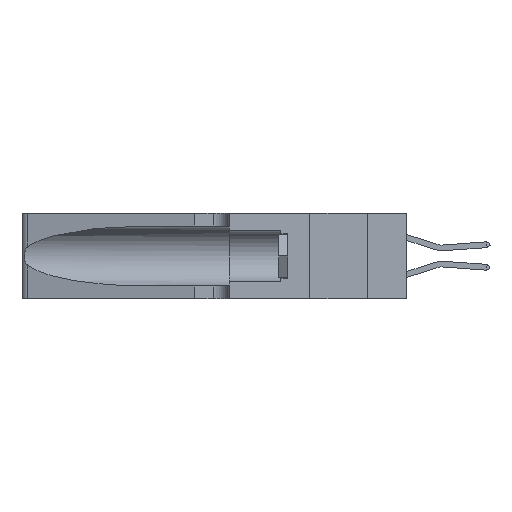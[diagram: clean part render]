
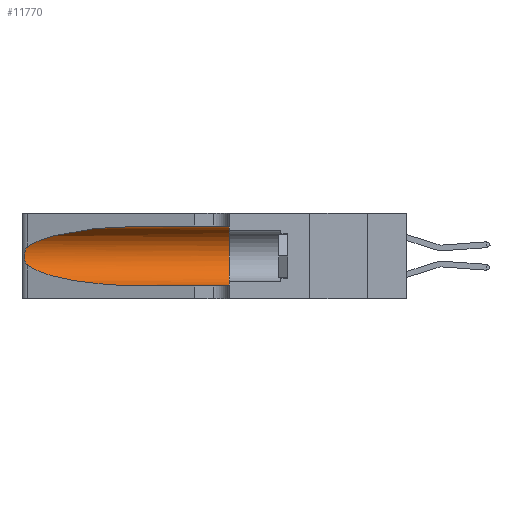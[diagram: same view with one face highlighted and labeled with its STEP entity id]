
A CAD part, left-side view. The second image highlights one B-rep face of the part: STEP entity #11770.
In plain terms, the highlighted cylindrical face has radius 3.308 mm (diameter 6.617 mm), a partial arc.
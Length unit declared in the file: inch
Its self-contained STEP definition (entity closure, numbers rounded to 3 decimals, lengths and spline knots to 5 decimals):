
#532 = AXIS2_PLACEMENT_3D ( 'NONE', #5945, #30028, #9462 ) ;
#824 = CARTESIAN_POINT ( 'NONE',  ( 0.25639, 1.23184, 0.21858 ) ) ;
#1131 = VERTEX_POINT ( 'NONE', #11829 ) ;
#1831 = DIRECTION ( 'NONE',  ( 0., 0., -1. ) ) ;
#1973 = VERTEX_POINT ( 'NONE', #43382 ) ;
#1997 = DIRECTION ( 'NONE',  ( 0., -1., 0. ) ) ;
#2877 = VECTOR ( 'NONE', #40002, 39.37008 ) ;
#3616 = B_SPLINE_CURVE_WITH_KNOTS ( 'NONE', 3,
 ( #18134, #38602, #824, #25039, #4360, #28454, #7872, #31913, #11397, #35346, #14853, #38744, #18292, #42131 ),
 .UNSPECIFIED., .F., .F.,
 ( 4, 2, 2, 2, 2, 2, 4 ),
 ( 0., 0.00027, 0.00053, 0.00107, 0.0016, 0.00187, 0.00214 ),
 .UNSPECIFIED. ) ;
#4360 = CARTESIAN_POINT ( 'NONE',  ( 0.25854, 1.2359, 0.20912 ) ) ;
#5945 = CARTESIAN_POINT ( 'NONE',  ( 0.1305, 0.35, 0.185 ) ) ;
#6686 = CARTESIAN_POINT ( 'NONE',  ( 0.25487, 1.22718, 0.14631 ) ) ;
#6868 = CARTESIAN_POINT ( 'NONE',  ( 0.1305, 0.72297, 0.31525 ) ) ;
#7448 = VERTEX_POINT ( 'NONE', #22350 ) ;
#7872 = CARTESIAN_POINT ( 'NONE',  ( 0.26075, 1.23896, 0.19203 ) ) ;
#8957 = EDGE_CURVE ( 'NONE', #12043, #1131, #30405, .T. ) ;
#9340 = VECTOR ( 'NONE', #41418, 39.37008 ) ;
#9462 = DIRECTION ( 'NONE',  ( 0., 0., 1. ) ) ;
#10227 = CARTESIAN_POINT ( 'NONE',  ( 0.18966, 0.96281, 0.05475 ) ) ;
#11397 = CARTESIAN_POINT ( 'NONE',  ( 0.26017, 1.23833, 0.17102 ) ) ;
#11628 = EDGE_CURVE ( 'NONE', #12043, #7448, #35634, .T. ) ;
#11770 = ADVANCED_FACE ( 'NONE', ( #26924 ), #43936, .F. ) ;
#11829 = CARTESIAN_POINT ( 'NONE',  ( 0.1305, 0.35, 0.31525 ) ) ;
#12043 = VERTEX_POINT ( 'NONE', #6868 ) ;
#14853 = CARTESIAN_POINT ( 'NONE',  ( 0.25789, 1.23486, 0.15765 ) ) ;
#15100 = CARTESIAN_POINT ( 'NONE',  ( 0.1305, 0.72297, 0.31525 ) ) ;
#17027 = CARTESIAN_POINT ( 'NONE',  ( 0.1305, 0.72297, 0.05475 ) ) ;
#17839 = VERTEX_POINT ( 'NONE', #20857 ) ;
#18134 = CARTESIAN_POINT ( 'NONE',  ( 0.25487, 1.22718, 0.22369 ) ) ;
#18237 = ORIENTED_EDGE ( 'NONE', *, *, #27362, .F. ) ;
#18292 = CARTESIAN_POINT ( 'NONE',  ( 0.25555, 1.22993, 0.14849 ) ) ;
#18500 = EDGE_CURVE ( 'NONE', #7448, #17839, #3616, .T. ) ;
#18524 = CARTESIAN_POINT ( 'NONE',  ( 0.18966, 0.96281, 0.31525 ) ) ;
#19537 = LINE ( 'NONE', #38019, #9340 ) ;
#20554 = AXIS2_PLACEMENT_3D ( 'NONE', #22712, #1997, #1831 ) ;
#20857 = CARTESIAN_POINT ( 'NONE',  ( 0.25487, 1.22718, 0.14631 ) ) ;
#21966 = CARTESIAN_POINT ( 'NONE',  ( 0.25487, 1.22718, 0.22369 ) ) ;
#22350 = CARTESIAN_POINT ( 'NONE',  ( 0.25487, 1.22718, 0.22369 ) ) ;
#22712 = CARTESIAN_POINT ( 'NONE',  ( 0.1305, 1.61858, 0.185 ) ) ;
#23768 = EDGE_CURVE ( 'NONE', #17839, #25146, #32357, .T. ) ;
#25039 = CARTESIAN_POINT ( 'NONE',  ( 0.25787, 1.23484, 0.2124 ) ) ;
#25146 = VERTEX_POINT ( 'NONE', #17027 ) ;
#25731 = ORIENTED_EDGE ( 'NONE', *, *, #11628, .T. ) ;
#26301 = ORIENTED_EDGE ( 'NONE', *, *, #32294, .T. ) ;
#26924 = FACE_OUTER_BOUND ( 'NONE', #38947, .T. ) ;
#27307 = CARTESIAN_POINT ( 'NONE',  ( 0.2373, 1.15595, 0.08982 ) ) ;
#27362 = EDGE_CURVE ( 'NONE', #1131, #1973, #38348, .T. ) ;
#28454 = CARTESIAN_POINT ( 'NONE',  ( 0.26018, 1.23835, 0.19895 ) ) ;
#30028 = DIRECTION ( 'NONE',  ( 0., 1., 0. ) ) ;
#30405 = LINE ( 'NONE', #33174, #2877 ) ;
#30590 = ORIENTED_EDGE ( 'NONE', *, *, #8957, .F. ) ;
#31913 = CARTESIAN_POINT ( 'NONE',  ( 0.26075, 1.23896, 0.178 ) ) ;
#32167 = ORIENTED_EDGE ( 'NONE', *, *, #23768, .T. ) ;
#32294 = EDGE_CURVE ( 'NONE', #25146, #1973, #19537, .T. ) ;
#32357 =( BOUNDED_CURVE ( )  B_SPLINE_CURVE ( 3, ( #6686, #27307, #10227, #34193 ),
 .UNSPECIFIED., .F., .F. ) 
 B_SPLINE_CURVE_WITH_KNOTS ( ( 4, 4 ),
 ( 3.44316, 4.71239 ),
 .UNSPECIFIED. ) 
 CURVE ( )  GEOMETRIC_REPRESENTATION_ITEM ( )  RATIONAL_B_SPLINE_CURVE ( ( 1., 0.87, 0.87, 1. ) ) 
 REPRESENTATION_ITEM ( '' )  );
#33174 = CARTESIAN_POINT ( 'NONE',  ( 0.1305, 1.61858, 0.31525 ) ) ;
#34193 = CARTESIAN_POINT ( 'NONE',  ( 0.1305, 0.72297, 0.05475 ) ) ;
#35346 = CARTESIAN_POINT ( 'NONE',  ( 0.25856, 1.23593, 0.16098 ) ) ;
#35634 =( BOUNDED_CURVE ( )  B_SPLINE_CURVE ( 3, ( #15100, #18524, #42384, #21966 ),
 .UNSPECIFIED., .F., .F. ) 
 B_SPLINE_CURVE_WITH_KNOTS ( ( 4, 4 ),
 ( 1.5708, 2.84003 ),
 .UNSPECIFIED. ) 
 CURVE ( )  GEOMETRIC_REPRESENTATION_ITEM ( )  RATIONAL_B_SPLINE_CURVE ( ( 1., 0.87, 0.87, 1. ) ) 
 REPRESENTATION_ITEM ( '' )  );
#37997 = ORIENTED_EDGE ( 'NONE', *, *, #18500, .T. ) ;
#38019 = CARTESIAN_POINT ( 'NONE',  ( 0.1305, 1.61858, 0.05475 ) ) ;
#38348 = CIRCLE ( 'NONE', #532, 0.13025 ) ;
#38602 = CARTESIAN_POINT ( 'NONE',  ( 0.25555, 1.22994, 0.2215 ) ) ;
#38744 = CARTESIAN_POINT ( 'NONE',  ( 0.25639, 1.23186, 0.15144 ) ) ;
#38947 = EDGE_LOOP ( 'NONE', ( #25731, #37997, #32167, #26301, #18237, #30590 ) ) ;
#40002 = DIRECTION ( 'NONE',  ( 0., -1., 0. ) ) ;
#41418 = DIRECTION ( 'NONE',  ( 0., -1., 0. ) ) ;
#42131 = CARTESIAN_POINT ( 'NONE',  ( 0.25487, 1.22718, 0.14631 ) ) ;
#42384 = CARTESIAN_POINT ( 'NONE',  ( 0.2373, 1.15595, 0.28018 ) ) ;
#43382 = CARTESIAN_POINT ( 'NONE',  ( 0.1305, 0.35, 0.05475 ) ) ;
#43936 = CYLINDRICAL_SURFACE ( 'NONE', #20554, 0.13025 ) ;
